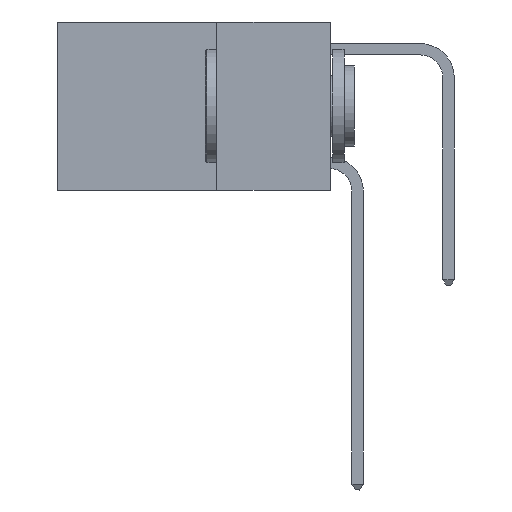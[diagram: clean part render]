
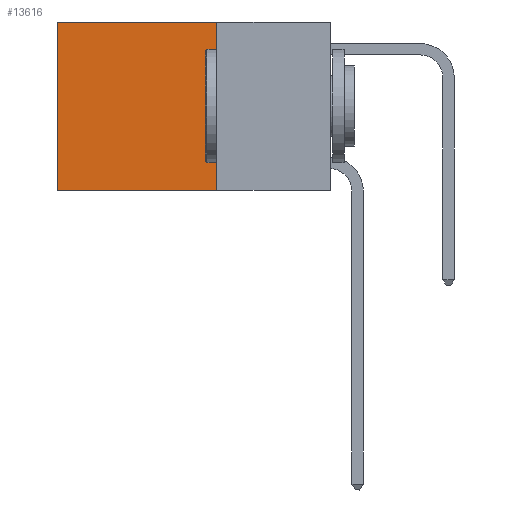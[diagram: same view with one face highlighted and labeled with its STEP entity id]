
A CAD part, left-side view. The second image highlights one B-rep face of the part: STEP entity #13616.
In plain terms, the highlighted planar face has unit normal (-1, 0, 0).
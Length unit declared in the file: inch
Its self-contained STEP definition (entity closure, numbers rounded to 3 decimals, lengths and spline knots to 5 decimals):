
#1280 = CARTESIAN_POINT ( 'NONE',  ( 0.2625, 0.25, 0. ) ) ;
#1299 = LINE ( 'NONE', #5821, #14908 ) ;
#3047 = LINE ( 'NONE', #1280, #9684 ) ;
#3200 = ORIENTED_EDGE ( 'NONE', *, *, #14754, .F. ) ;
#3314 = CARTESIAN_POINT ( 'NONE',  ( 0.2625, 0.25, 0. ) ) ;
#3748 = EDGE_CURVE ( 'NONE', #8190, #12412, #3047, .T. ) ;
#4238 = VECTOR ( 'NONE', #8053, 39.37008 ) ;
#4560 = DIRECTION ( 'NONE',  ( 0., 1., 0. ) ) ;
#5261 = VERTEX_POINT ( 'NONE', #12275 ) ;
#5636 = ORIENTED_EDGE ( 'NONE', *, *, #9479, .T. ) ;
#5731 = PLANE ( 'NONE',  #15654 ) ;
#5779 = DIRECTION ( 'NONE',  ( 1., 0., 0. ) ) ;
#5821 = CARTESIAN_POINT ( 'NONE',  ( 0.2625, 0.25, -0.37 ) ) ;
#7358 = VECTOR ( 'NONE', #4560, 39.37008 ) ;
#7413 = VERTEX_POINT ( 'NONE', #12155 ) ;
#7735 = LINE ( 'NONE', #11910, #4238 ) ;
#8053 = DIRECTION ( 'NONE',  ( 0., 0., -1. ) ) ;
#8190 = VERTEX_POINT ( 'NONE', #3314 ) ;
#9479 = EDGE_CURVE ( 'NONE', #8190, #7413, #14169, .T. ) ;
#9684 = VECTOR ( 'NONE', #15709, 39.37008 ) ;
#9786 = EDGE_LOOP ( 'NONE', ( #15796, #3200, #13472, #5636 ) ) ;
#10036 = EDGE_CURVE ( 'NONE', #7413, #5261, #7735, .T. ) ;
#11315 = CARTESIAN_POINT ( 'NONE',  ( 0.2625, 0.25, -0.37 ) ) ;
#11910 = CARTESIAN_POINT ( 'NONE',  ( 0.2625, 0.6, 0. ) ) ;
#12155 = CARTESIAN_POINT ( 'NONE',  ( 0.2625, 0.6, 0. ) ) ;
#12275 = CARTESIAN_POINT ( 'NONE',  ( 0.2625, 0.6, -0.37 ) ) ;
#12412 = VERTEX_POINT ( 'NONE', #11315 ) ;
#13152 = FACE_OUTER_BOUND ( 'NONE', #9786, .T. ) ;
#13459 = CARTESIAN_POINT ( 'NONE',  ( 0.2625, 0.25, 0. ) ) ;
#13472 = ORIENTED_EDGE ( 'NONE', *, *, #3748, .F. ) ;
#13494 = DIRECTION ( 'NONE',  ( 0., 1., 0. ) ) ;
#13580 = CARTESIAN_POINT ( 'NONE',  ( 0.2625, 0.25, 0. ) ) ;
#13616 = ADVANCED_FACE ( 'NONE', ( #13152 ), #5731, .F. ) ;
#14169 = LINE ( 'NONE', #13580, #7358 ) ;
#14732 = DIRECTION ( 'NONE',  ( 0., 0., -1. ) ) ;
#14754 = EDGE_CURVE ( 'NONE', #12412, #5261, #1299, .T. ) ;
#14908 = VECTOR ( 'NONE', #13494, 39.37008 ) ;
#15654 = AXIS2_PLACEMENT_3D ( 'NONE', #13459, #5779, #14732 ) ;
#15709 = DIRECTION ( 'NONE',  ( 0., 0., -1. ) ) ;
#15796 = ORIENTED_EDGE ( 'NONE', *, *, #10036, .T. ) ;
